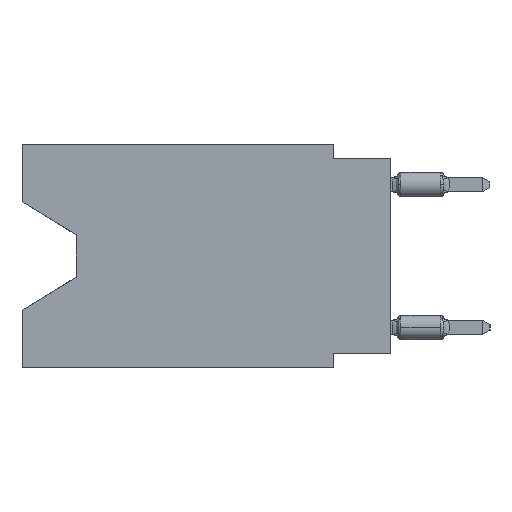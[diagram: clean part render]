
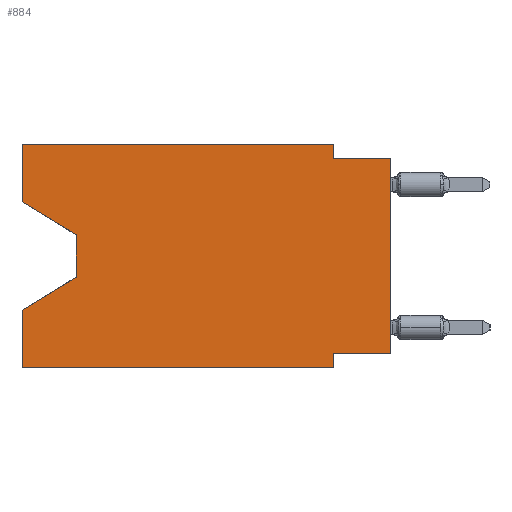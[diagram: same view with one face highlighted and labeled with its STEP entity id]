
A CAD part, left-side view. The second image highlights one B-rep face of the part: STEP entity #884.
In plain terms, the highlighted planar face has unit normal (-1, 0, 0).
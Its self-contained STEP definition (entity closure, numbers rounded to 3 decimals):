
#62 = VECTOR ( 'NONE', #31289, 1000. ) ;
#705 = EDGE_CURVE ( 'NONE', #41414, #4549, #6055, .T. ) ;
#884 = ADVANCED_FACE ( 'NONE', ( #29358 ), #25940, .F. ) ;
#1024 = CARTESIAN_POINT ( 'NONE',  ( 0., 2.54, -0.635 ) ) ;
#1735 = DIRECTION ( 'NONE',  ( 0., 0.855, -0.519 ) ) ;
#1786 = DIRECTION ( 'NONE',  ( 0., -1., 0. ) ) ;
#2822 = LINE ( 'NONE', #28575, #22913 ) ;
#3163 = VECTOR ( 'NONE', #1786, 1000. ) ;
#3418 = DIRECTION ( 'NONE',  ( 0., -1., 0. ) ) ;
#3744 = VERTEX_POINT ( 'NONE', #39054 ) ;
#3821 = CARTESIAN_POINT ( 'NONE',  ( 0., 16.383, 0. ) ) ;
#4549 = VERTEX_POINT ( 'NONE', #32324 ) ;
#5324 = ORIENTED_EDGE ( 'NONE', *, *, #18390, .F. ) ;
#6055 = LINE ( 'NONE', #9692, #18000 ) ;
#6185 = DIRECTION ( 'NONE',  ( 0., 0., -1. ) ) ;
#6553 = EDGE_CURVE ( 'NONE', #17279, #37823, #2822, .T. ) ;
#6942 = DIRECTION ( 'NONE',  ( 0., 0., 1. ) ) ;
#7491 = CARTESIAN_POINT ( 'NONE',  ( 0., 0., -9.271 ) ) ;
#8625 = VECTOR ( 'NONE', #22022, 1000. ) ;
#9692 = CARTESIAN_POINT ( 'NONE',  ( 0., 16.383, -2.546 ) ) ;
#10609 = VERTEX_POINT ( 'NONE', #1024 ) ;
#10699 = VECTOR ( 'NONE', #6185, 1000. ) ;
#11333 = ORIENTED_EDGE ( 'NONE', *, *, #22632, .F. ) ;
#11813 = LINE ( 'NONE', #3821, #8625 ) ;
#12178 = CARTESIAN_POINT ( 'NONE',  ( 0., 2.54, 0. ) ) ;
#12581 = CARTESIAN_POINT ( 'NONE',  ( 0., 16.383, -9.906 ) ) ;
#12824 = DIRECTION ( 'NONE',  ( 0., -1., 0. ) ) ;
#13326 = CARTESIAN_POINT ( 'NONE',  ( 0., 0., -9.271 ) ) ;
#13713 = CARTESIAN_POINT ( 'NONE',  ( 0., 2.54, -9.271 ) ) ;
#14056 = EDGE_LOOP ( 'NONE', ( #44926, #36715, #20259, #36664, #17988, #43031, #39088, #15505, #11333, #24934, #5324, #43008 ) ) ;
#15255 = DIRECTION ( 'NONE',  ( 1., 0., 0. ) ) ;
#15302 = EDGE_CURVE ( 'NONE', #17279, #25817, #31773, .T. ) ;
#15380 = EDGE_CURVE ( 'NONE', #22961, #20024, #38819, .T. ) ;
#15505 = ORIENTED_EDGE ( 'NONE', *, *, #15380, .T. ) ;
#15567 = EDGE_CURVE ( 'NONE', #41414, #3744, #11813, .T. ) ;
#15872 = CARTESIAN_POINT ( 'NONE',  ( 0., 16.383, -9.906 ) ) ;
#17279 = VERTEX_POINT ( 'NONE', #15872 ) ;
#17988 = ORIENTED_EDGE ( 'NONE', *, *, #15302, .T. ) ;
#18000 = VECTOR ( 'NONE', #29126, 1000. ) ;
#18390 = EDGE_CURVE ( 'NONE', #3744, #30981, #19522, .T. ) ;
#18870 = EDGE_CURVE ( 'NONE', #46613, #37823, #20193, .T. ) ;
#19522 = LINE ( 'NONE', #31424, #3163 ) ;
#20024 = VERTEX_POINT ( 'NONE', #42803 ) ;
#20193 = LINE ( 'NONE', #35023, #27001 ) ;
#20259 = ORIENTED_EDGE ( 'NONE', *, *, #18870, .T. ) ;
#21317 = CARTESIAN_POINT ( 'NONE',  ( 0., 16.383, -7.36 ) ) ;
#22022 = DIRECTION ( 'NONE',  ( 0., 0., 1. ) ) ;
#22105 = CARTESIAN_POINT ( 'NONE',  ( 0., 0., -0.635 ) ) ;
#22537 = CARTESIAN_POINT ( 'NONE',  ( 0., 16.383, 0. ) ) ;
#22632 = EDGE_CURVE ( 'NONE', #10609, #20024, #37402, .T. ) ;
#22913 = VECTOR ( 'NONE', #6942, 1000. ) ;
#22961 = VERTEX_POINT ( 'NONE', #7491 ) ;
#23115 = LINE ( 'NONE', #42554, #41524 ) ;
#23607 = EDGE_CURVE ( 'NONE', #4549, #46613, #23115, .T. ) ;
#24075 = DIRECTION ( 'NONE',  ( 0., 0., -1. ) ) ;
#24085 = EDGE_CURVE ( 'NONE', #22961, #47867, #35683, .T. ) ;
#24934 = ORIENTED_EDGE ( 'NONE', *, *, #25507, .F. ) ;
#25507 = EDGE_CURVE ( 'NONE', #30981, #10609, #34676, .T. ) ;
#25817 = VERTEX_POINT ( 'NONE', #29070 ) ;
#25940 = PLANE ( 'NONE',  #38978 ) ;
#26853 = CARTESIAN_POINT ( 'NONE',  ( 0., 16.383, -2.546 ) ) ;
#27001 = VECTOR ( 'NONE', #1735, 1000. ) ;
#28575 = CARTESIAN_POINT ( 'NONE',  ( 0., 16.383, 0. ) ) ;
#29070 = CARTESIAN_POINT ( 'NONE',  ( 0., 2.54, -9.906 ) ) ;
#29126 = DIRECTION ( 'NONE',  ( 0., -0.855, -0.519 ) ) ;
#29358 = FACE_OUTER_BOUND ( 'NONE', #14056, .T. ) ;
#29920 = VECTOR ( 'NONE', #46369, 1000. ) ;
#30812 = CARTESIAN_POINT ( 'NONE',  ( 0., 0., 0. ) ) ;
#30981 = VERTEX_POINT ( 'NONE', #12178 ) ;
#31289 = DIRECTION ( 'NONE',  ( 0., 0., 1. ) ) ;
#31424 = CARTESIAN_POINT ( 'NONE',  ( 0., 16.383, 0. ) ) ;
#31773 = LINE ( 'NONE', #12581, #45830 ) ;
#32324 = CARTESIAN_POINT ( 'NONE',  ( 0., 13.97, -4.013 ) ) ;
#33652 = VECTOR ( 'NONE', #38315, 1000. ) ;
#34676 = LINE ( 'NONE', #41967, #33652 ) ;
#34851 = LINE ( 'NONE', #38973, #10699 ) ;
#35023 = CARTESIAN_POINT ( 'NONE',  ( 0., 13.97, -5.893 ) ) ;
#35683 = LINE ( 'NONE', #13326, #29920 ) ;
#36664 = ORIENTED_EDGE ( 'NONE', *, *, #6553, .F. ) ;
#36715 = ORIENTED_EDGE ( 'NONE', *, *, #23607, .T. ) ;
#37402 = LINE ( 'NONE', #22105, #45332 ) ;
#37823 = VERTEX_POINT ( 'NONE', #21317 ) ;
#38315 = DIRECTION ( 'NONE',  ( 0., 0., -1. ) ) ;
#38819 = LINE ( 'NONE', #30812, #62 ) ;
#38973 = CARTESIAN_POINT ( 'NONE',  ( 0., 2.54, -9.906 ) ) ;
#38978 = AXIS2_PLACEMENT_3D ( 'NONE', #22537, #15255, #41018 ) ;
#39054 = CARTESIAN_POINT ( 'NONE',  ( 0., 16.383, 0. ) ) ;
#39060 = EDGE_CURVE ( 'NONE', #47867, #25817, #34851, .T. ) ;
#39088 = ORIENTED_EDGE ( 'NONE', *, *, #24085, .F. ) ;
#41018 = DIRECTION ( 'NONE',  ( 0., 0., -1. ) ) ;
#41414 = VERTEX_POINT ( 'NONE', #26853 ) ;
#41524 = VECTOR ( 'NONE', #24075, 1000. ) ;
#41967 = CARTESIAN_POINT ( 'NONE',  ( 0., 2.54, 0. ) ) ;
#42554 = CARTESIAN_POINT ( 'NONE',  ( 0., 13.97, -4.013 ) ) ;
#42803 = CARTESIAN_POINT ( 'NONE',  ( 0., 0., -0.635 ) ) ;
#43008 = ORIENTED_EDGE ( 'NONE', *, *, #15567, .F. ) ;
#43031 = ORIENTED_EDGE ( 'NONE', *, *, #39060, .F. ) ;
#43103 = CARTESIAN_POINT ( 'NONE',  ( 0., 13.97, -5.893 ) ) ;
#44926 = ORIENTED_EDGE ( 'NONE', *, *, #705, .T. ) ;
#45332 = VECTOR ( 'NONE', #3418, 1000. ) ;
#45830 = VECTOR ( 'NONE', #12824, 1000. ) ;
#46369 = DIRECTION ( 'NONE',  ( 0., 1., 0. ) ) ;
#46613 = VERTEX_POINT ( 'NONE', #43103 ) ;
#47867 = VERTEX_POINT ( 'NONE', #13713 ) ;
